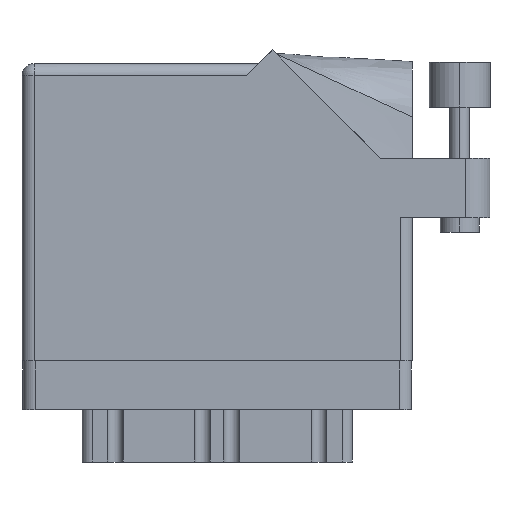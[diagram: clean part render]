
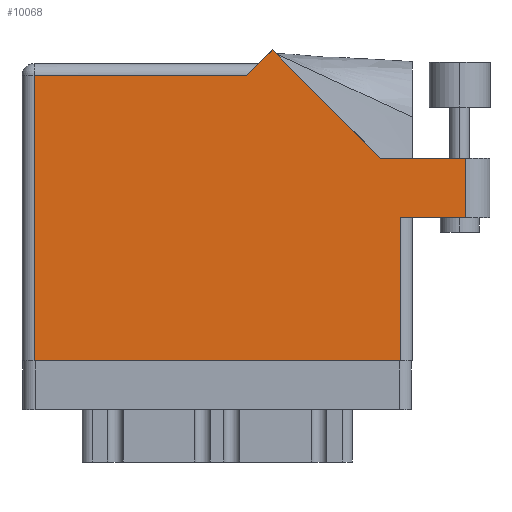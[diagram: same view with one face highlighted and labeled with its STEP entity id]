
A CAD part, front view. The second image highlights one B-rep face of the part: STEP entity #10068.
In plain terms, the highlighted face is planar.
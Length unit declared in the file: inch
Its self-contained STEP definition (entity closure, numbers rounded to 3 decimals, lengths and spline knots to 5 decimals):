
#656 = CARTESIAN_POINT ( 'NONE',  ( 2.285, 0.737, 0. ) ) ;
#1225 = CARTESIAN_POINT ( 'NONE',  ( 0., 1.468, 0. ) ) ;
#1520 = VECTOR ( 'NONE', #10466, 39.37008 ) ;
#2221 = VERTEX_POINT ( 'NONE', #13593 ) ;
#2227 = CARTESIAN_POINT ( 'NONE',  ( 2.41, 1.044, 0. ) ) ;
#3340 = VERTEX_POINT ( 'NONE', #12279 ) ;
#4137 = EDGE_CURVE ( 'NONE', #13324, #21296, #20396, .T. ) ;
#4266 = AXIS2_PLACEMENT_3D ( 'NONE', #16257, #21882, #12821 ) ;
#4604 = EDGE_LOOP ( 'NONE', ( #5148, #26582, #10718, #21453, #9357, #23747, #20451, #5648, #9538 ) ) ;
#5048 = LINE ( 'NONE', #28900, #14968 ) ;
#5148 = ORIENTED_EDGE ( 'NONE', *, *, #21395, .T. ) ;
#5278 = VECTOR ( 'NONE', #11758, 39.37008 ) ;
#5648 = ORIENTED_EDGE ( 'NONE', *, *, #33236, .T. ) ;
#6622 = VECTOR ( 'NONE', #19777, 39.37008 ) ;
#6995 = VECTOR ( 'NONE', #28800, 39.37008 ) ;
#8101 = CARTESIAN_POINT ( 'NONE',  ( 1.155, 1.468, 0. ) ) ;
#9357 = ORIENTED_EDGE ( 'NONE', *, *, #28593, .T. ) ;
#9538 = ORIENTED_EDGE ( 'NONE', *, *, #24331, .T. ) ;
#9563 = CARTESIAN_POINT ( 'NONE',  ( 1.948, 0.737, 0. ) ) ;
#9858 = CARTESIAN_POINT ( 'NONE',  ( 2.01, 0.737, 0. ) ) ;
#9860 = CARTESIAN_POINT ( 'NONE',  ( 2.285, 1.044, 0. ) ) ;
#10068 = ADVANCED_FACE ( 'NONE', ( #21057 ), #34365, .F. ) ;
#10466 = DIRECTION ( 'NONE',  ( -1., 0., 0. ) ) ;
#10718 = ORIENTED_EDGE ( 'NONE', *, *, #25373, .T. ) ;
#11537 = EDGE_CURVE ( 'NONE', #19835, #16947, #14368, .T. ) ;
#11758 = DIRECTION ( 'NONE',  ( -1., 0., 0. ) ) ;
#12039 = CARTESIAN_POINT ( 'NONE',  ( 1.84442, 1.044, 0. ) ) ;
#12279 = CARTESIAN_POINT ( 'NONE',  ( 1.28771, 1.60071, 0. ) ) ;
#12497 = LINE ( 'NONE', #9858, #6995 ) ;
#12821 = DIRECTION ( 'NONE',  ( -1., 0., 0. ) ) ;
#13324 = VERTEX_POINT ( 'NONE', #656 ) ;
#13593 = CARTESIAN_POINT ( 'NONE',  ( 1.948, 0., 0. ) ) ;
#13867 = DIRECTION ( 'NONE',  ( 1., 0., 0. ) ) ;
#14368 = LINE ( 'NONE', #1225, #5278 ) ;
#14577 = VERTEX_POINT ( 'NONE', #19470 ) ;
#14968 = VECTOR ( 'NONE', #21013, 39.37008 ) ;
#15059 = LINE ( 'NONE', #23135, #32508 ) ;
#15805 = CARTESIAN_POINT ( 'NONE',  ( 0.062, 1.468, 0. ) ) ;
#16257 = CARTESIAN_POINT ( 'NONE',  ( 0., 1.53, 0. ) ) ;
#16603 = VERTEX_POINT ( 'NONE', #34627 ) ;
#16947 = VERTEX_POINT ( 'NONE', #15805 ) ;
#17978 = VERTEX_POINT ( 'NONE', #9563 ) ;
#19470 = CARTESIAN_POINT ( 'NONE',  ( 0.062, 0., 0. ) ) ;
#19777 = DIRECTION ( 'NONE',  ( 0., 1., 0. ) ) ;
#19835 = VERTEX_POINT ( 'NONE', #8101 ) ;
#20396 = LINE ( 'NONE', #9860, #22333 ) ;
#20451 = ORIENTED_EDGE ( 'NONE', *, *, #25324, .T. ) ;
#20501 = DIRECTION ( 'NONE',  ( -0.707, -0.707, 0. ) ) ;
#20566 = DIRECTION ( 'NONE',  ( 0., 1., 0. ) ) ;
#21013 = DIRECTION ( 'NONE',  ( 0., -1., 0. ) ) ;
#21057 = FACE_OUTER_BOUND ( 'NONE', #4604, .T. ) ;
#21258 = CARTESIAN_POINT ( 'NONE',  ( 0., 0., 0. ) ) ;
#21296 = VERTEX_POINT ( 'NONE', #28284 ) ;
#21395 = EDGE_CURVE ( 'NONE', #17978, #13324, #12497, .T. ) ;
#21453 = ORIENTED_EDGE ( 'NONE', *, *, #25522, .T. ) ;
#21882 = DIRECTION ( 'NONE',  ( 0., 0., -1. ) ) ;
#22333 = VECTOR ( 'NONE', #20566, 39.37008 ) ;
#23135 = CARTESIAN_POINT ( 'NONE',  ( 1.217, 1.53, 0. ) ) ;
#23747 = ORIENTED_EDGE ( 'NONE', *, *, #11537, .T. ) ;
#23804 = VECTOR ( 'NONE', #13867, 39.37008 ) ;
#24331 = EDGE_CURVE ( 'NONE', #2221, #17978, #25385, .T. ) ;
#25032 = LINE ( 'NONE', #12039, #30654 ) ;
#25324 = EDGE_CURVE ( 'NONE', #16947, #14577, #5048, .T. ) ;
#25373 = EDGE_CURVE ( 'NONE', #21296, #16603, #28576, .T. ) ;
#25385 = LINE ( 'NONE', #28178, #6622 ) ;
#25522 = EDGE_CURVE ( 'NONE', #16603, #3340, #25032, .T. ) ;
#25549 = DIRECTION ( 'NONE',  ( -0.707, 0.707, 0. ) ) ;
#26582 = ORIENTED_EDGE ( 'NONE', *, *, #4137, .T. ) ;
#28178 = CARTESIAN_POINT ( 'NONE',  ( 1.948, 0.737, 0. ) ) ;
#28284 = CARTESIAN_POINT ( 'NONE',  ( 2.285, 1.044, 0. ) ) ;
#28576 = LINE ( 'NONE', #2227, #1520 ) ;
#28593 = EDGE_CURVE ( 'NONE', #3340, #19835, #15059, .T. ) ;
#28800 = DIRECTION ( 'NONE',  ( 1., 0., 0. ) ) ;
#28900 = CARTESIAN_POINT ( 'NONE',  ( 0.062, 0., 0. ) ) ;
#30654 = VECTOR ( 'NONE', #25549, 39.37008 ) ;
#31940 = LINE ( 'NONE', #21258, #23804 ) ;
#32508 = VECTOR ( 'NONE', #20501, 39.37008 ) ;
#33236 = EDGE_CURVE ( 'NONE', #14577, #2221, #31940, .T. ) ;
#34365 = PLANE ( 'NONE',  #4266 ) ;
#34627 = CARTESIAN_POINT ( 'NONE',  ( 1.84442, 1.044, 0. ) ) ;
